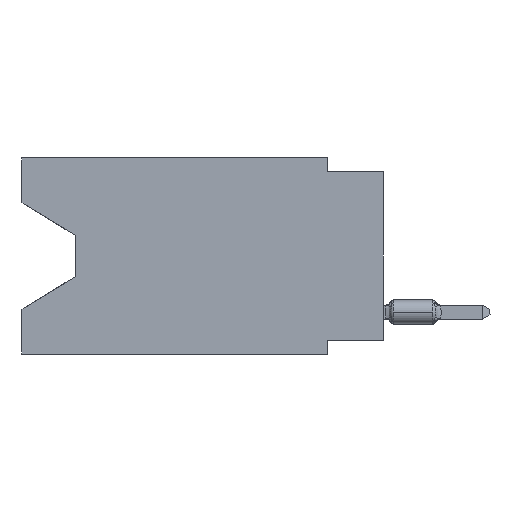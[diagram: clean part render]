
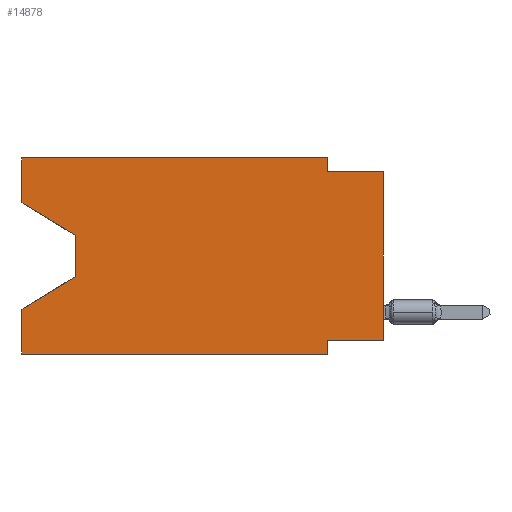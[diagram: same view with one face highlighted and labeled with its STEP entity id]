
A CAD part, left-side view. The second image highlights one B-rep face of the part: STEP entity #14878.
In plain terms, the highlighted planar face has unit normal (-1, 0, 0).
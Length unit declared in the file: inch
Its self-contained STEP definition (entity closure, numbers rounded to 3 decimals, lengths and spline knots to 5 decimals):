
#257 = LINE ( 'NONE', #4730, #17430 ) ;
#425 = DIRECTION ( 'NONE',  ( 1., 0., 0. ) ) ;
#513 = CARTESIAN_POINT ( 'NONE',  ( 0., 0.645, 0. ) ) ;
#845 = EDGE_CURVE ( 'NONE', #18817, #18902, #16632, .T. ) ;
#1301 = DIRECTION ( 'NONE',  ( 0., 0., -1. ) ) ;
#1320 = LINE ( 'NONE', #8872, #18580 ) ;
#1793 = DIRECTION ( 'NONE',  ( 0., -1., 0. ) ) ;
#1919 = DIRECTION ( 'NONE',  ( 0., 0., -1. ) ) ;
#2020 = CARTESIAN_POINT ( 'NONE',  ( 0., 0.1, -0.325 ) ) ;
#2133 = CARTESIAN_POINT ( 'NONE',  ( 0., 0.1, -0.025 ) ) ;
#2490 = VECTOR ( 'NONE', #11729, 39.37008 ) ;
#2523 = CARTESIAN_POINT ( 'NONE',  ( 0., 0., -0.025 ) ) ;
#2603 = EDGE_CURVE ( 'NONE', #11113, #3837, #6297, .T. ) ;
#2606 = VECTOR ( 'NONE', #15559, 39.37008 ) ;
#2629 = ORIENTED_EDGE ( 'NONE', *, *, #2603, .F. ) ;
#3296 = EDGE_CURVE ( 'NONE', #13035, #5953, #3958, .T. ) ;
#3399 = FACE_OUTER_BOUND ( 'NONE', #4165, .T. ) ;
#3430 = CARTESIAN_POINT ( 'NONE',  ( 0., 0.645, -0.35 ) ) ;
#3525 = CARTESIAN_POINT ( 'NONE',  ( 0., 0.55, -0.138 ) ) ;
#3837 = VERTEX_POINT ( 'NONE', #2020 ) ;
#3958 = LINE ( 'NONE', #16412, #4528 ) ;
#4165 = EDGE_LOOP ( 'NONE', ( #18661, #8642, #16448, #10478, #8719, #5138, #2629, #18808, #9691, #9268, #13896, #17087 ) ) ;
#4428 = CARTESIAN_POINT ( 'NONE',  ( 0., 0.1, -0.35 ) ) ;
#4528 = VECTOR ( 'NONE', #8835, 39.37008 ) ;
#4598 = CARTESIAN_POINT ( 'NONE',  ( 0., 0., -0.325 ) ) ;
#4625 = DIRECTION ( 'NONE',  ( 0., 0., 1. ) ) ;
#4730 = CARTESIAN_POINT ( 'NONE',  ( 0., 0., 0. ) ) ;
#5051 = DIRECTION ( 'NONE',  ( 0., 0.855, -0.519 ) ) ;
#5059 = EDGE_CURVE ( 'NONE', #6029, #17350, #1320, .T. ) ;
#5138 = ORIENTED_EDGE ( 'NONE', *, *, #9628, .F. ) ;
#5245 = EDGE_CURVE ( 'NONE', #13035, #9962, #12750, .T. ) ;
#5645 = CARTESIAN_POINT ( 'NONE',  ( 0., 0.645, 0. ) ) ;
#5953 = VERTEX_POINT ( 'NONE', #3525 ) ;
#6029 = VERTEX_POINT ( 'NONE', #3430 ) ;
#6216 = DIRECTION ( 'NONE',  ( 0., 0., -1. ) ) ;
#6297 = LINE ( 'NONE', #4598, #2606 ) ;
#6669 = DIRECTION ( 'NONE',  ( 0., 0., 1. ) ) ;
#6784 = VECTOR ( 'NONE', #6669, 39.37008 ) ;
#6916 = CARTESIAN_POINT ( 'NONE',  ( 0., 0.55, -0.212 ) ) ;
#7151 = LINE ( 'NONE', #14836, #14700 ) ;
#7441 = EDGE_CURVE ( 'NONE', #15890, #18200, #17565, .T. ) ;
#8180 = CARTESIAN_POINT ( 'NONE',  ( 0., 0.645, 0. ) ) ;
#8536 = LINE ( 'NONE', #5645, #2490 ) ;
#8642 = ORIENTED_EDGE ( 'NONE', *, *, #15085, .T. ) ;
#8719 = ORIENTED_EDGE ( 'NONE', *, *, #5059, .T. ) ;
#8835 = DIRECTION ( 'NONE',  ( 0., -0.855, -0.519 ) ) ;
#8872 = CARTESIAN_POINT ( 'NONE',  ( 0., 0.645, -0.35 ) ) ;
#8965 = AXIS2_PLACEMENT_3D ( 'NONE', #15555, #425, #1919 ) ;
#9058 = VERTEX_POINT ( 'NONE', #14730 ) ;
#9068 = DIRECTION ( 'NONE',  ( 0., -1., 0. ) ) ;
#9268 = ORIENTED_EDGE ( 'NONE', *, *, #11249, .F. ) ;
#9430 = VECTOR ( 'NONE', #5051, 39.37008 ) ;
#9472 = PLANE ( 'NONE',  #8965 ) ;
#9628 = EDGE_CURVE ( 'NONE', #3837, #17350, #10234, .T. ) ;
#9691 = ORIENTED_EDGE ( 'NONE', *, *, #845, .F. ) ;
#9868 = DIRECTION ( 'NONE',  ( 0., -1., 0. ) ) ;
#9962 = VERTEX_POINT ( 'NONE', #16857 ) ;
#10066 = LINE ( 'NONE', #8180, #12701 ) ;
#10234 = LINE ( 'NONE', #16511, #17395 ) ;
#10303 = CARTESIAN_POINT ( 'NONE',  ( 0., 0.645, -0.08025 ) ) ;
#10478 = ORIENTED_EDGE ( 'NONE', *, *, #18066, .F. ) ;
#10707 = LINE ( 'NONE', #12404, #13295 ) ;
#10941 = VECTOR ( 'NONE', #1793, 39.37008 ) ;
#11113 = VERTEX_POINT ( 'NONE', #15076 ) ;
#11248 = EDGE_CURVE ( 'NONE', #11113, #18902, #257, .T. ) ;
#11249 = EDGE_CURVE ( 'NONE', #9058, #18817, #10707, .T. ) ;
#11729 = DIRECTION ( 'NONE',  ( 0., 0., 1. ) ) ;
#12404 = CARTESIAN_POINT ( 'NONE',  ( 0., 0.1, 0. ) ) ;
#12701 = VECTOR ( 'NONE', #9868, 39.37008 ) ;
#12750 = LINE ( 'NONE', #513, #6784 ) ;
#13035 = VERTEX_POINT ( 'NONE', #10303 ) ;
#13295 = VECTOR ( 'NONE', #6216, 39.37008 ) ;
#13321 = CARTESIAN_POINT ( 'NONE',  ( 0., 0.645, -0.26975 ) ) ;
#13896 = ORIENTED_EDGE ( 'NONE', *, *, #19243, .F. ) ;
#14700 = VECTOR ( 'NONE', #1301, 39.37008 ) ;
#14730 = CARTESIAN_POINT ( 'NONE',  ( 0., 0.1, 0. ) ) ;
#14836 = CARTESIAN_POINT ( 'NONE',  ( 0., 0.55, -0.138 ) ) ;
#14878 = ADVANCED_FACE ( 'NONE', ( #3399 ), #9472, .F. ) ;
#15076 = CARTESIAN_POINT ( 'NONE',  ( 0., 0., -0.325 ) ) ;
#15085 = EDGE_CURVE ( 'NONE', #5953, #15890, #7151, .T. ) ;
#15555 = CARTESIAN_POINT ( 'NONE',  ( 0., 0.645, 0. ) ) ;
#15559 = DIRECTION ( 'NONE',  ( 0., 1., 0. ) ) ;
#15890 = VERTEX_POINT ( 'NONE', #6916 ) ;
#16063 = CARTESIAN_POINT ( 'NONE',  ( 0., 0.55, -0.212 ) ) ;
#16210 = DIRECTION ( 'NONE',  ( 0., 0., -1. ) ) ;
#16412 = CARTESIAN_POINT ( 'NONE',  ( 0., 0.645, -0.08025 ) ) ;
#16448 = ORIENTED_EDGE ( 'NONE', *, *, #7441, .T. ) ;
#16511 = CARTESIAN_POINT ( 'NONE',  ( 0., 0.1, -0.35 ) ) ;
#16632 = LINE ( 'NONE', #16832, #10941 ) ;
#16832 = CARTESIAN_POINT ( 'NONE',  ( 0., 0., -0.025 ) ) ;
#16857 = CARTESIAN_POINT ( 'NONE',  ( 0., 0.645, 0. ) ) ;
#17087 = ORIENTED_EDGE ( 'NONE', *, *, #5245, .F. ) ;
#17350 = VERTEX_POINT ( 'NONE', #4428 ) ;
#17395 = VECTOR ( 'NONE', #16210, 39.37008 ) ;
#17430 = VECTOR ( 'NONE', #4625, 39.37008 ) ;
#17565 = LINE ( 'NONE', #16063, #9430 ) ;
#18066 = EDGE_CURVE ( 'NONE', #6029, #18200, #8536, .T. ) ;
#18200 = VERTEX_POINT ( 'NONE', #13321 ) ;
#18580 = VECTOR ( 'NONE', #9068, 39.37008 ) ;
#18661 = ORIENTED_EDGE ( 'NONE', *, *, #3296, .T. ) ;
#18808 = ORIENTED_EDGE ( 'NONE', *, *, #11248, .T. ) ;
#18817 = VERTEX_POINT ( 'NONE', #2133 ) ;
#18902 = VERTEX_POINT ( 'NONE', #2523 ) ;
#19243 = EDGE_CURVE ( 'NONE', #9962, #9058, #10066, .T. ) ;
